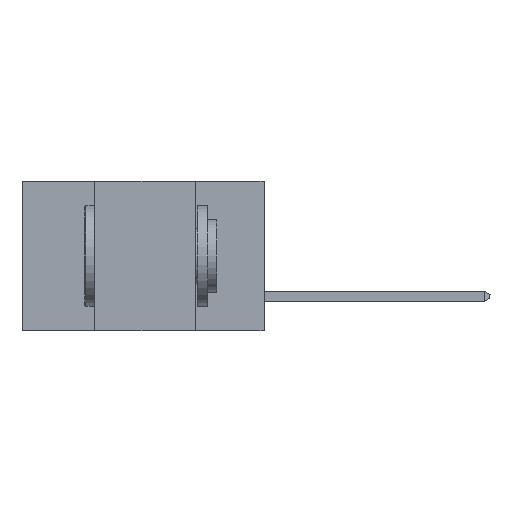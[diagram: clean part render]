
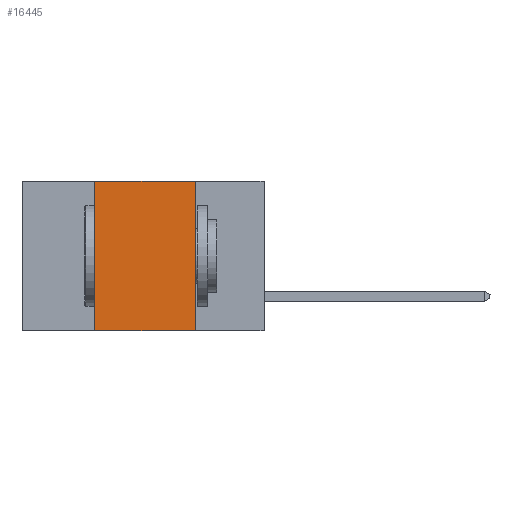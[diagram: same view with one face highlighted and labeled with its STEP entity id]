
A CAD part, left-side view. The second image highlights one B-rep face of the part: STEP entity #16445.
In plain terms, the highlighted planar face has unit normal (-1, 0, 0).
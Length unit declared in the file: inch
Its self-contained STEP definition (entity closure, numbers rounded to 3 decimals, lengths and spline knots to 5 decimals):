
#85 = LINE ( 'NONE', #5333, #2294 ) ;
#793 = ORIENTED_EDGE ( 'NONE', *, *, #13202, .F. ) ;
#854 = DIRECTION ( 'NONE',  ( 0., -1., 0. ) ) ;
#983 = AXIS2_PLACEMENT_3D ( 'NONE', #4354, #4266, #15263 ) ;
#1450 = ORIENTED_EDGE ( 'NONE', *, *, #6838, .F. ) ;
#2294 = VECTOR ( 'NONE', #11010, 39.37008 ) ;
#2395 = VERTEX_POINT ( 'NONE', #3432 ) ;
#2968 = VERTEX_POINT ( 'NONE', #9095 ) ;
#3122 = ORIENTED_EDGE ( 'NONE', *, *, #13482, .F. ) ;
#3432 = CARTESIAN_POINT ( 'NONE',  ( 0., 0.42, -0.37 ) ) ;
#4121 = EDGE_CURVE ( 'NONE', #2395, #6426, #8932, .T. ) ;
#4266 = DIRECTION ( 'NONE',  ( 1., 0., 0. ) ) ;
#4354 = CARTESIAN_POINT ( 'NONE',  ( 0., 0.6, 0. ) ) ;
#4380 = VERTEX_POINT ( 'NONE', #10982 ) ;
#5333 = CARTESIAN_POINT ( 'NONE',  ( 0., 0.17, -0.37 ) ) ;
#5853 = ORIENTED_EDGE ( 'NONE', *, *, #4121, .T. ) ;
#5870 = CARTESIAN_POINT ( 'NONE',  ( 0., 0.6, -0.37 ) ) ;
#6426 = VERTEX_POINT ( 'NONE', #9517 ) ;
#6838 = EDGE_CURVE ( 'NONE', #4380, #6426, #85, .T. ) ;
#6913 = EDGE_LOOP ( 'NONE', ( #1450, #3122, #793, #5853 ) ) ;
#7442 = VECTOR ( 'NONE', #7490, 39.37008 ) ;
#7490 = DIRECTION ( 'NONE',  ( 0., -1., 0. ) ) ;
#8256 = PLANE ( 'NONE',  #983 ) ;
#8651 = DIRECTION ( 'NONE',  ( 0., 0., 1. ) ) ;
#8932 = LINE ( 'NONE', #5870, #7442 ) ;
#9095 = CARTESIAN_POINT ( 'NONE',  ( 0., 0.42, 0. ) ) ;
#9335 = VECTOR ( 'NONE', #8651, 39.37008 ) ;
#9517 = CARTESIAN_POINT ( 'NONE',  ( 0., 0.17, -0.37 ) ) ;
#10338 = LINE ( 'NONE', #15822, #13916 ) ;
#10982 = CARTESIAN_POINT ( 'NONE',  ( 0., 0.17, 0. ) ) ;
#11010 = DIRECTION ( 'NONE',  ( 0., 0., -1. ) ) ;
#11347 = LINE ( 'NONE', #12768, #9335 ) ;
#12768 = CARTESIAN_POINT ( 'NONE',  ( 0., 0.42, -0.37 ) ) ;
#13202 = EDGE_CURVE ( 'NONE', #2395, #2968, #11347, .T. ) ;
#13482 = EDGE_CURVE ( 'NONE', #2968, #4380, #10338, .T. ) ;
#13804 = FACE_OUTER_BOUND ( 'NONE', #6913, .T. ) ;
#13916 = VECTOR ( 'NONE', #854, 39.37008 ) ;
#15263 = DIRECTION ( 'NONE',  ( 0., 0., -1. ) ) ;
#15822 = CARTESIAN_POINT ( 'NONE',  ( 0., 0.6, 0. ) ) ;
#16445 = ADVANCED_FACE ( 'NONE', ( #13804 ), #8256, .F. ) ;
